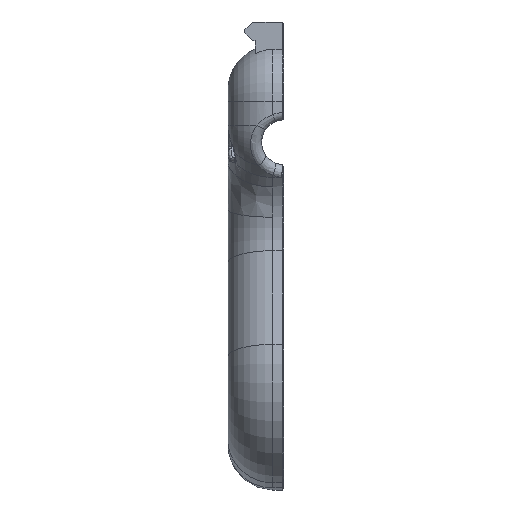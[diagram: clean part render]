
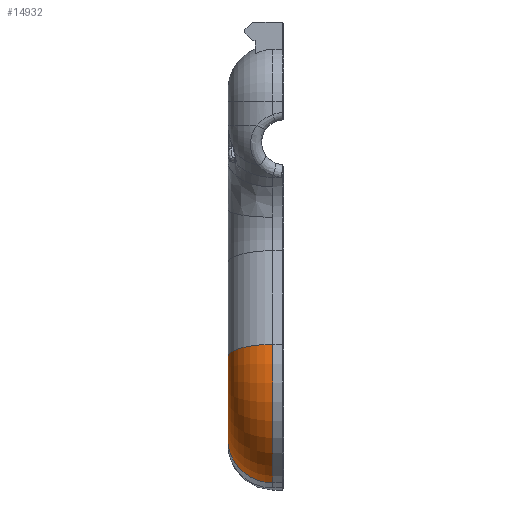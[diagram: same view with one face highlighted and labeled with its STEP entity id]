
A CAD part, left-side view. The second image highlights one B-rep face of the part: STEP entity #14932.
In plain terms, the highlighted toroidal (fillet/blend) face has major radius 18 mm and minor radius 12 mm.
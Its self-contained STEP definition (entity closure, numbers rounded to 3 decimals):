
#3864 = CYLINDRICAL_SURFACE('',#3865,30.);
#3865 = AXIS2_PLACEMENT_3D('',#3866,#3867,#3868);
#3866 = CARTESIAN_POINT('',(-25.893,-15.,-79.431));
#3867 = DIRECTION('',(0.,1.,0.));
#3868 = DIRECTION('',(-0.276,0.,-0.961));
#8954 = VERTEX_POINT('',#8955);
#8955 = CARTESIAN_POINT('',(-34.162,3.,-108.269));
#8992 = CYLINDRICAL_SURFACE('',#8993,12.);
#8993 = AXIS2_PLACEMENT_3D('',#8994,#8995,#8996);
#8994 = CARTESIAN_POINT('',(-26.048,3.,-98.112));
#8995 = DIRECTION('',(-0.961,0.,0.276));
#8996 = DIRECTION('',(-0.276,0.,-0.961));
#9010 = VERTEX_POINT('',#9011);
#9011 = CARTESIAN_POINT('',(-54.731,3.,-71.162));
#9032 = EDGE_CURVE('',#8954,#9010,#9033,.T.);
#9033 = SURFACE_CURVE('',#9034,(#9039,#9046),.PCURVE_S1.);
#9034 = CIRCLE('',#9035,30.);
#9035 = AXIS2_PLACEMENT_3D('',#9036,#9037,#9038);
#9036 = CARTESIAN_POINT('',(-25.893,3.,-79.431));
#9037 = DIRECTION('',(0.,1.,0.));
#9038 = DIRECTION('',(-0.276,0.,-0.961));
#9039 = PCURVE('',#3864,#9040);
#9040 = DEFINITIONAL_REPRESENTATION('',(#9041),#9045);
#9041 = LINE('',#9042,#9043);
#9042 = CARTESIAN_POINT('',(0.,18.));
#9043 = VECTOR('',#9044,1.);
#9044 = DIRECTION('',(1.,0.));
#9045 = ( GEOMETRIC_REPRESENTATION_CONTEXT(2) 
PARAMETRIC_REPRESENTATION_CONTEXT() REPRESENTATION_CONTEXT('2D SPACE',''
  ) );
#9046 = PCURVE('',#9047,#9052);
#9047 = TOROIDAL_SURFACE('',#9048,18.,12.);
#9048 = AXIS2_PLACEMENT_3D('',#9049,#9050,#9051);
#9049 = CARTESIAN_POINT('',(-25.893,3.,-79.431));
#9050 = DIRECTION('',(0.,1.,0.));
#9051 = DIRECTION('',(-0.276,0.,-0.961));
#9052 = DEFINITIONAL_REPRESENTATION('',(#9053),#9057);
#9053 = LINE('',#9054,#9055);
#9054 = CARTESIAN_POINT('',(0.,0.));
#9055 = VECTOR('',#9056,1.);
#9056 = DIRECTION('',(1.,0.));
#9057 = ( GEOMETRIC_REPRESENTATION_CONTEXT(2) 
PARAMETRIC_REPRESENTATION_CONTEXT() REPRESENTATION_CONTEXT('2D SPACE',''
  ) );
#9101 = CYLINDRICAL_SURFACE('',#9102,12.);
#9102 = AXIS2_PLACEMENT_3D('',#9103,#9104,#9105);
#9103 = CARTESIAN_POINT('',(-43.196,3.,-74.47));
#9104 = DIRECTION('',(0.276,0.,0.961));
#9105 = DIRECTION('',(-0.961,0.,0.276));
#14804 = PLANE('',#14805);
#14805 = AXIS2_PLACEMENT_3D('',#14806,#14807,#14808);
#14806 = CARTESIAN_POINT('',(10.936,15.,-32.273));
#14807 = DIRECTION('',(0.,1.,0.));
#14808 = DIRECTION('',(0.,0.,1.));
#14890 = VERTEX_POINT('',#14891);
#14891 = CARTESIAN_POINT('',(-30.855,15.,-96.734));
#14912 = EDGE_CURVE('',#8954,#14890,#14913,.T.);
#14913 = SURFACE_CURVE('',#14914,(#14919,#14925),.PCURVE_S1.);
#14914 = CIRCLE('',#14915,12.);
#14915 = AXIS2_PLACEMENT_3D('',#14916,#14917,#14918);
#14916 = CARTESIAN_POINT('',(-30.855,3.,-96.734));
#14917 = DIRECTION('',(0.961,0.,-0.276));
#14918 = DIRECTION('',(-0.276,0.,-0.961));
#14919 = PCURVE('',#8992,#14920);
#14920 = DEFINITIONAL_REPRESENTATION('',(#14921),#14924);
#14921 = B_SPLINE_CURVE_WITH_KNOTS('',1,(#14922,#14923),.UNSPECIFIED.,
  .F.,.F.,(2,2),(0.,1.571),.PIECEWISE_BEZIER_KNOTS.);
#14922 = CARTESIAN_POINT('',(0.,5.));
#14923 = CARTESIAN_POINT('',(-1.571,5.));
#14924 = ( GEOMETRIC_REPRESENTATION_CONTEXT(2) 
PARAMETRIC_REPRESENTATION_CONTEXT() REPRESENTATION_CONTEXT('2D SPACE',''
  ) );
#14925 = PCURVE('',#9047,#14926);
#14926 = DEFINITIONAL_REPRESENTATION('',(#14927),#14930);
#14927 = B_SPLINE_CURVE_WITH_KNOTS('',1,(#14928,#14929),.UNSPECIFIED.,
  .F.,.F.,(2,2),(0.,1.571),.PIECEWISE_BEZIER_KNOTS.);
#14928 = CARTESIAN_POINT('',(0.,0.));
#14929 = CARTESIAN_POINT('',(0.,1.571));
#14930 = ( GEOMETRIC_REPRESENTATION_CONTEXT(2) 
PARAMETRIC_REPRESENTATION_CONTEXT() REPRESENTATION_CONTEXT('2D SPACE',''
  ) );
#14932 = ADVANCED_FACE('',(#14933),#9047,.T.);
#14933 = FACE_BOUND('',#14934,.T.);
#14934 = EDGE_LOOP('',(#14935,#14936,#14937,#14959));
#14935 = ORIENTED_EDGE('',*,*,#14912,.F.);
#14936 = ORIENTED_EDGE('',*,*,#9032,.T.);
#14937 = ORIENTED_EDGE('',*,*,#14938,.T.);
#14938 = EDGE_CURVE('',#9010,#14939,#14941,.T.);
#14939 = VERTEX_POINT('',#14940);
#14940 = CARTESIAN_POINT('',(-43.196,15.,-74.47));
#14941 = SURFACE_CURVE('',#14942,(#14947,#14953),.PCURVE_S1.);
#14942 = CIRCLE('',#14943,12.);
#14943 = AXIS2_PLACEMENT_3D('',#14944,#14945,#14946);
#14944 = CARTESIAN_POINT('',(-43.196,3.,-74.47));
#14945 = DIRECTION('',(-0.276,0.,-0.961));
#14946 = DIRECTION('',(-0.961,0.,0.276));
#14947 = PCURVE('',#9047,#14948);
#14948 = DEFINITIONAL_REPRESENTATION('',(#14949),#14952);
#14949 = B_SPLINE_CURVE_WITH_KNOTS('',1,(#14950,#14951),.UNSPECIFIED.,
  .F.,.F.,(2,2),(0.,1.571),.PIECEWISE_BEZIER_KNOTS.);
#14950 = CARTESIAN_POINT('',(1.571,0.));
#14951 = CARTESIAN_POINT('',(1.571,1.571));
#14952 = ( GEOMETRIC_REPRESENTATION_CONTEXT(2) 
PARAMETRIC_REPRESENTATION_CONTEXT() REPRESENTATION_CONTEXT('2D SPACE',''
  ) );
#14953 = PCURVE('',#9101,#14954);
#14954 = DEFINITIONAL_REPRESENTATION('',(#14955),#14958);
#14955 = B_SPLINE_CURVE_WITH_KNOTS('',1,(#14956,#14957),.UNSPECIFIED.,
  .F.,.F.,(2,2),(0.,1.571),.PIECEWISE_BEZIER_KNOTS.);
#14956 = CARTESIAN_POINT('',(0.,0.));
#14957 = CARTESIAN_POINT('',(-1.571,0.));
#14958 = ( GEOMETRIC_REPRESENTATION_CONTEXT(2) 
PARAMETRIC_REPRESENTATION_CONTEXT() REPRESENTATION_CONTEXT('2D SPACE',''
  ) );
#14959 = ORIENTED_EDGE('',*,*,#14960,.F.);
#14960 = EDGE_CURVE('',#14890,#14939,#14961,.T.);
#14961 = SURFACE_CURVE('',#14962,(#14967,#14974),.PCURVE_S1.);
#14962 = CIRCLE('',#14963,18.);
#14963 = AXIS2_PLACEMENT_3D('',#14964,#14965,#14966);
#14964 = CARTESIAN_POINT('',(-25.893,15.,-79.431));
#14965 = DIRECTION('',(0.,1.,0.));
#14966 = DIRECTION('',(-0.276,0.,-0.961));
#14967 = PCURVE('',#9047,#14968);
#14968 = DEFINITIONAL_REPRESENTATION('',(#14969),#14973);
#14969 = LINE('',#14970,#14971);
#14970 = CARTESIAN_POINT('',(0.,1.571));
#14971 = VECTOR('',#14972,1.);
#14972 = DIRECTION('',(1.,0.));
#14973 = ( GEOMETRIC_REPRESENTATION_CONTEXT(2) 
PARAMETRIC_REPRESENTATION_CONTEXT() REPRESENTATION_CONTEXT('2D SPACE',''
  ) );
#14974 = PCURVE('',#14804,#14975);
#14975 = DEFINITIONAL_REPRESENTATION('',(#14976),#14980);
#14976 = CIRCLE('',#14977,18.);
#14977 = AXIS2_PLACEMENT_2D('',#14978,#14979);
#14978 = CARTESIAN_POINT('',(-47.158,-36.829));
#14979 = DIRECTION('',(-0.961,-0.276));
#14980 = ( GEOMETRIC_REPRESENTATION_CONTEXT(2) 
PARAMETRIC_REPRESENTATION_CONTEXT() REPRESENTATION_CONTEXT('2D SPACE',''
  ) );
